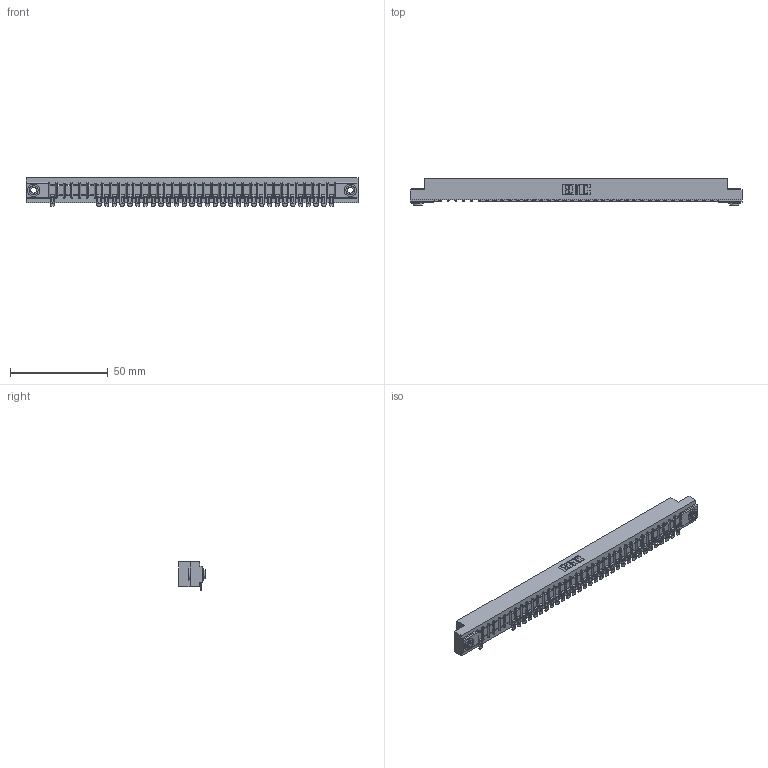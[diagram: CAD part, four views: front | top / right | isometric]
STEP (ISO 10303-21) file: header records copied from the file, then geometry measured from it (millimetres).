
FILE_DESCRIPTION (( 'STEP AP203' ), '1' );
FILE_NAME ('357-037-554-103.STEP', '2018-08-10T08:05:00', ( '' ), ( '' ), 'SwSTEP 2.0', 'SolidWorks 2016', '' );
FILE_SCHEMA (( 'CONFIG_CONTROL_DESIGN' ));
Length unit declared in the file: inch
Products named in the file (4): 357-037-554-103; 307 Part_.156 Dia Mounting Holes; 307-290-002_554; 345-250-002_345-250-002-102
Assembly tree (35 placements, depth 2):
  357-037-554-103
    307 Part_.156 Dia Mounting Holes
    307-290-002_554  x32
    345-250-002_345-250-002-102  x2
Bounding box: 169.62 x 13.36 x 14.52 mm (x, y, z)
Volume: 17982.5 mm3; surface area: 21946.6 mm2
Topology: 35 solids, 35 shells, 2900 faces, 8851 edges, 5794 vertices
Faces by surface type: plane 1626, cylinder 1190, sphere 76, cone 8
Entity records: 34206 total; most frequent: CARTESIAN_POINT 5770, ORIENTED_EDGE 5756, DIRECTION 5624, EDGE_CURVE 2878, LINE 2188, VECTOR 2188, VERTEX_POINT 1864, AXIS2_PLACEMENT_3D 1718
